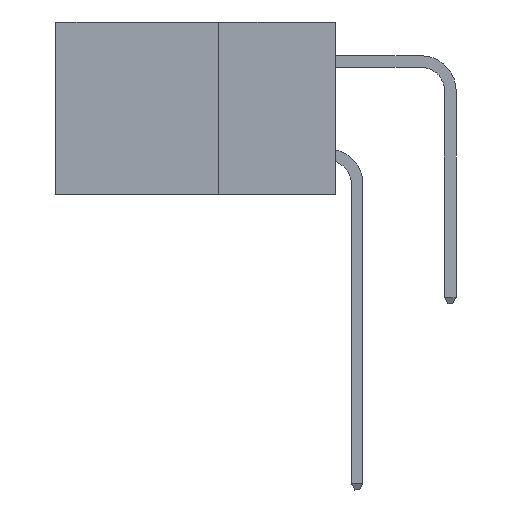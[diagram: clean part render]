
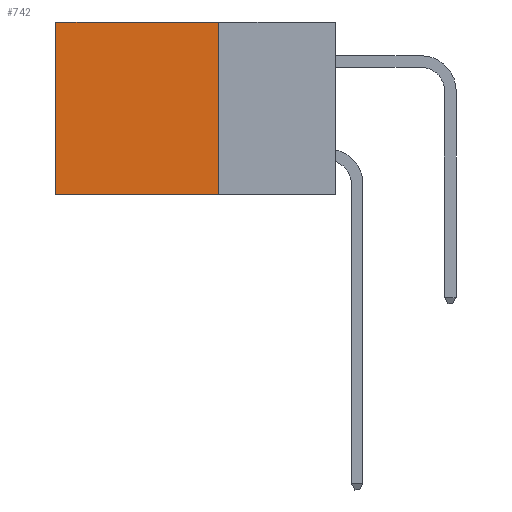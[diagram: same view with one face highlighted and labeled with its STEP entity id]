
A CAD part, left-side view. The second image highlights one B-rep face of the part: STEP entity #742.
In plain terms, the highlighted planar face has unit normal (-1, 0, 0).
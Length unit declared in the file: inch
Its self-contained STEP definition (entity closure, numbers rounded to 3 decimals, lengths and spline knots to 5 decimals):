
#332 = CARTESIAN_POINT ( 'NONE',  ( 0.2875, 0.6, 0. ) ) ;
#742 = ADVANCED_FACE ( 'NONE', ( #10195 ), #7931, .F. ) ;
#958 = DIRECTION ( 'NONE',  ( 0., 0., -1. ) ) ;
#1023 = EDGE_CURVE ( 'NONE', #2994, #6268, #5003, .T. ) ;
#1497 = VECTOR ( 'NONE', #12873, 39.37008 ) ;
#1560 = EDGE_CURVE ( 'NONE', #11666, #2249, #10002, .T. ) ;
#1664 = VECTOR ( 'NONE', #958, 39.37008 ) ;
#1688 = ORIENTED_EDGE ( 'NONE', *, *, #2406, .T. ) ;
#1819 = ORIENTED_EDGE ( 'NONE', *, *, #1560, .F. ) ;
#1869 = ORIENTED_EDGE ( 'NONE', *, *, #5430, .F. ) ;
#1923 = ORIENTED_EDGE ( 'NONE', *, *, #1023, .T. ) ;
#2130 = VECTOR ( 'NONE', #6940, 39.37008 ) ;
#2249 = VERTEX_POINT ( 'NONE', #3012 ) ;
#2406 = EDGE_CURVE ( 'NONE', #6268, #2249, #9796, .T. ) ;
#2784 = DIRECTION ( 'NONE',  ( 0., 0., -1. ) ) ;
#2811 = EDGE_LOOP ( 'NONE', ( #1688, #1819, #1869, #1923 ) ) ;
#2994 = VERTEX_POINT ( 'NONE', #3739 ) ;
#3012 = CARTESIAN_POINT ( 'NONE',  ( 0.2875, 0.6, -0.37 ) ) ;
#3109 = CARTESIAN_POINT ( 'NONE',  ( 0.2875, 0.25, 0. ) ) ;
#3252 = LINE ( 'NONE', #3109, #5684 ) ;
#3508 = CARTESIAN_POINT ( 'NONE',  ( 0.2875, 0.25, 0. ) ) ;
#3739 = CARTESIAN_POINT ( 'NONE',  ( 0.2875, 0.25, 0. ) ) ;
#5003 = LINE ( 'NONE', #3508, #2130 ) ;
#5430 = EDGE_CURVE ( 'NONE', #2994, #11666, #3252, .T. ) ;
#5684 = VECTOR ( 'NONE', #2784, 39.37008 ) ;
#6182 = AXIS2_PLACEMENT_3D ( 'NONE', #7890, #7830, #7496 ) ;
#6268 = VERTEX_POINT ( 'NONE', #332 ) ;
#6301 = CARTESIAN_POINT ( 'NONE',  ( 0.2875, 0.25, -0.37 ) ) ;
#6940 = DIRECTION ( 'NONE',  ( 0., 1., 0. ) ) ;
#7496 = DIRECTION ( 'NONE',  ( 0., 0., -1. ) ) ;
#7830 = DIRECTION ( 'NONE',  ( 1., 0., 0. ) ) ;
#7890 = CARTESIAN_POINT ( 'NONE',  ( 0.2875, 0.25, 0. ) ) ;
#7931 = PLANE ( 'NONE',  #6182 ) ;
#9247 = CARTESIAN_POINT ( 'NONE',  ( 0.2875, 0.6, 0. ) ) ;
#9796 = LINE ( 'NONE', #9247, #1664 ) ;
#10002 = LINE ( 'NONE', #12705, #1497 ) ;
#10195 = FACE_OUTER_BOUND ( 'NONE', #2811, .T. ) ;
#11666 = VERTEX_POINT ( 'NONE', #6301 ) ;
#12705 = CARTESIAN_POINT ( 'NONE',  ( 0.2875, 0.25, -0.37 ) ) ;
#12873 = DIRECTION ( 'NONE',  ( 0., 1., 0. ) ) ;
